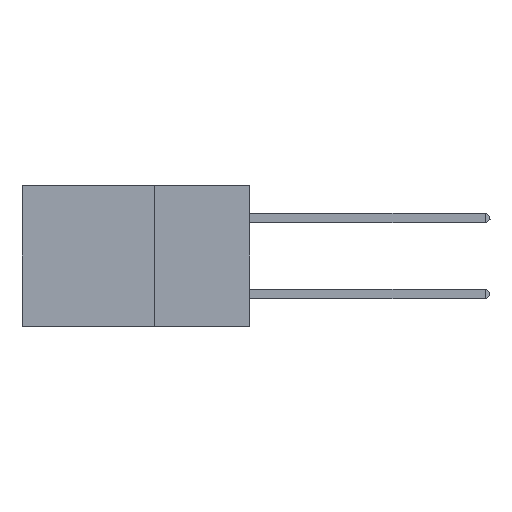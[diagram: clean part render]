
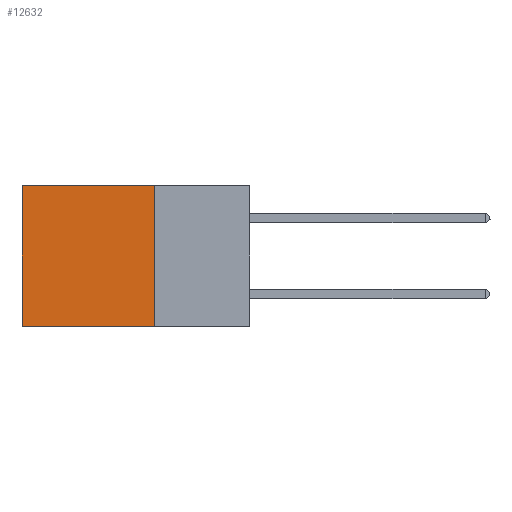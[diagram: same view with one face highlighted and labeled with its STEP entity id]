
A CAD part, left-side view. The second image highlights one B-rep face of the part: STEP entity #12632.
In plain terms, the highlighted planar face has unit normal (-1, 0, 0).
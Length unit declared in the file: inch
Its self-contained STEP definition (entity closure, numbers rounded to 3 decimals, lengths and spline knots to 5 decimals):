
#544 = LINE ( 'NONE', #1025, #2109 ) ;
#767 = ORIENTED_EDGE ( 'NONE', *, *, #23792, .T. ) ;
#1025 = CARTESIAN_POINT ( 'NONE',  ( 0.2875, 0.25, 0. ) ) ;
#2109 = VECTOR ( 'NONE', #15477, 39.37008 ) ;
#2768 = ORIENTED_EDGE ( 'NONE', *, *, #20184, .F. ) ;
#2941 = DIRECTION ( 'NONE',  ( 0., 1., 0. ) ) ;
#3811 = DIRECTION ( 'NONE',  ( 0., 0., -1. ) ) ;
#5471 = DIRECTION ( 'NONE',  ( 1., 0., 0. ) ) ;
#6843 = CARTESIAN_POINT ( 'NONE',  ( 0.2875, 0.6, -0.37 ) ) ;
#8235 = LINE ( 'NONE', #25669, #16145 ) ;
#8300 = LINE ( 'NONE', #13446, #19768 ) ;
#10500 = CARTESIAN_POINT ( 'NONE',  ( 0.2875, 0.6, 0. ) ) ;
#10746 = AXIS2_PLACEMENT_3D ( 'NONE', #28540, #5471, #23069 ) ;
#11014 = ORIENTED_EDGE ( 'NONE', *, *, #29505, .F. ) ;
#12632 = ADVANCED_FACE ( 'NONE', ( #30872 ), #29926, .F. ) ;
#13446 = CARTESIAN_POINT ( 'NONE',  ( 0.2875, 0.25, -0.37 ) ) ;
#13810 = VERTEX_POINT ( 'NONE', #6843 ) ;
#14945 = VERTEX_POINT ( 'NONE', #25162 ) ;
#15477 = DIRECTION ( 'NONE',  ( 0., 0., -1. ) ) ;
#16145 = VECTOR ( 'NONE', #2941, 39.37008 ) ;
#16235 = EDGE_CURVE ( 'NONE', #18829, #13810, #23584, .T. ) ;
#17545 = ORIENTED_EDGE ( 'NONE', *, *, #16235, .T. ) ;
#18092 = DIRECTION ( 'NONE',  ( 0., 1., 0. ) ) ;
#18829 = VERTEX_POINT ( 'NONE', #10500 ) ;
#19768 = VECTOR ( 'NONE', #18092, 39.37008 ) ;
#20184 = EDGE_CURVE ( 'NONE', #14945, #13810, #8300, .T. ) ;
#21848 = VERTEX_POINT ( 'NONE', #27368 ) ;
#22935 = CARTESIAN_POINT ( 'NONE',  ( 0.2875, 0.6, 0. ) ) ;
#23069 = DIRECTION ( 'NONE',  ( 0., 0., -1. ) ) ;
#23584 = LINE ( 'NONE', #22935, #26793 ) ;
#23792 = EDGE_CURVE ( 'NONE', #21848, #18829, #8235, .T. ) ;
#25162 = CARTESIAN_POINT ( 'NONE',  ( 0.2875, 0.25, -0.37 ) ) ;
#25669 = CARTESIAN_POINT ( 'NONE',  ( 0.2875, 0.25, 0. ) ) ;
#26793 = VECTOR ( 'NONE', #3811, 39.37008 ) ;
#27368 = CARTESIAN_POINT ( 'NONE',  ( 0.2875, 0.25, 0. ) ) ;
#28540 = CARTESIAN_POINT ( 'NONE',  ( 0.2875, 0.25, 0. ) ) ;
#29505 = EDGE_CURVE ( 'NONE', #21848, #14945, #544, .T. ) ;
#29926 = PLANE ( 'NONE',  #10746 ) ;
#30872 = FACE_OUTER_BOUND ( 'NONE', #32383, .T. ) ;
#32383 = EDGE_LOOP ( 'NONE', ( #17545, #2768, #11014, #767 ) ) ;
